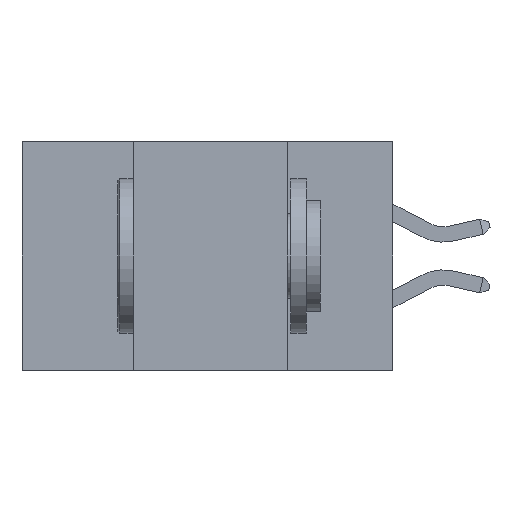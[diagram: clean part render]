
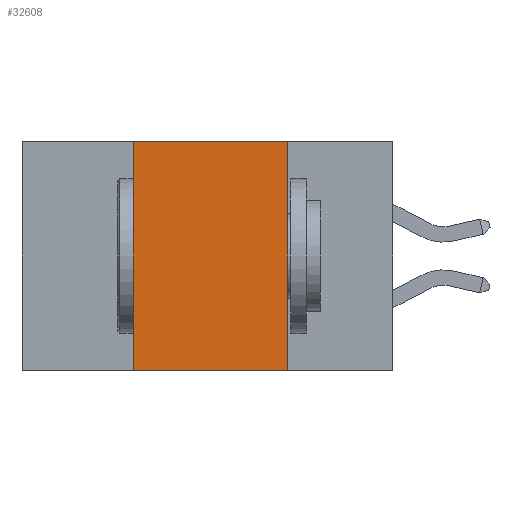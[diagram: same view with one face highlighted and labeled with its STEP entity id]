
A CAD part, left-side view. The second image highlights one B-rep face of the part: STEP entity #32608.
In plain terms, the highlighted planar face has unit normal (-1, 0, 0).
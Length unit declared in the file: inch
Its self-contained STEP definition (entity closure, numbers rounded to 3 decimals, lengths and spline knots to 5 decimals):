
#1119 = ORIENTED_EDGE ( 'NONE', *, *, #39357, .T. ) ;
#2064 = EDGE_CURVE ( 'NONE', #19710, #17247, #11782, .T. ) ;
#4725 = VECTOR ( 'NONE', #20893, 39.37008 ) ;
#6675 = ORIENTED_EDGE ( 'NONE', *, *, #34340, .F. ) ;
#6849 = LINE ( 'NONE', #10185, #23837 ) ;
#9267 = LINE ( 'NONE', #37215, #34528 ) ;
#10185 = CARTESIAN_POINT ( 'NONE',  ( 0., 0.17, 0. ) ) ;
#11579 = CARTESIAN_POINT ( 'NONE',  ( 0., 0.17, 0. ) ) ;
#11782 = LINE ( 'NONE', #29937, #33029 ) ;
#12444 = FACE_OUTER_BOUND ( 'NONE', #28556, .T. ) ;
#12488 = CARTESIAN_POINT ( 'NONE',  ( 0., 0.6, 0. ) ) ;
#13299 = LINE ( 'NONE', #17681, #4725 ) ;
#16404 = CARTESIAN_POINT ( 'NONE',  ( 0., 0.42, 0. ) ) ;
#17008 = CARTESIAN_POINT ( 'NONE',  ( 0., 0.17, -0.37 ) ) ;
#17247 = VERTEX_POINT ( 'NONE', #11579 ) ;
#17681 = CARTESIAN_POINT ( 'NONE',  ( 0., 0.42, 0. ) ) ;
#18092 = CARTESIAN_POINT ( 'NONE',  ( 0., 0.42, -0.37 ) ) ;
#18349 = DIRECTION ( 'NONE',  ( 0., -1., 0. ) ) ;
#18900 = DIRECTION ( 'NONE',  ( 1., 0., 0. ) ) ;
#19710 = VERTEX_POINT ( 'NONE', #16404 ) ;
#20622 = DIRECTION ( 'NONE',  ( 0., -1., 0. ) ) ;
#20893 = DIRECTION ( 'NONE',  ( 0., 0., 1. ) ) ;
#23651 = VERTEX_POINT ( 'NONE', #18092 ) ;
#23837 = VECTOR ( 'NONE', #32304, 39.37008 ) ;
#25089 = ORIENTED_EDGE ( 'NONE', *, *, #2064, .F. ) ;
#27229 = EDGE_CURVE ( 'NONE', #17247, #27362, #6849, .T. ) ;
#27362 = VERTEX_POINT ( 'NONE', #17008 ) ;
#28556 = EDGE_LOOP ( 'NONE', ( #38868, #25089, #6675, #1119 ) ) ;
#29937 = CARTESIAN_POINT ( 'NONE',  ( 0., 0.6, 0. ) ) ;
#32304 = DIRECTION ( 'NONE',  ( 0., 0., -1. ) ) ;
#32608 = ADVANCED_FACE ( 'NONE', ( #12444 ), #40750, .F. ) ;
#33029 = VECTOR ( 'NONE', #20622, 39.37008 ) ;
#34340 = EDGE_CURVE ( 'NONE', #23651, #19710, #13299, .T. ) ;
#34528 = VECTOR ( 'NONE', #18349, 39.37008 ) ;
#37215 = CARTESIAN_POINT ( 'NONE',  ( 0., 0.6, -0.37 ) ) ;
#38861 = AXIS2_PLACEMENT_3D ( 'NONE', #12488, #18900, #40881 ) ;
#38868 = ORIENTED_EDGE ( 'NONE', *, *, #27229, .F. ) ;
#39357 = EDGE_CURVE ( 'NONE', #23651, #27362, #9267, .T. ) ;
#40750 = PLANE ( 'NONE',  #38861 ) ;
#40881 = DIRECTION ( 'NONE',  ( 0., 0., -1. ) ) ;
